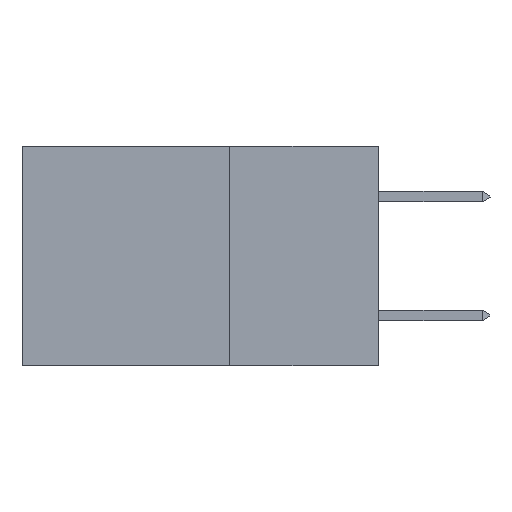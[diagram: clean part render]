
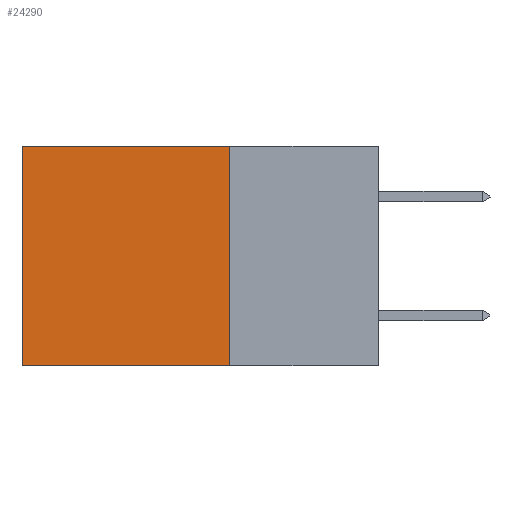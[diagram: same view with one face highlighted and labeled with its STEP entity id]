
A CAD part, left-side view. The second image highlights one B-rep face of the part: STEP entity #24290.
In plain terms, the highlighted planar face has unit normal (-1, 0, 0).
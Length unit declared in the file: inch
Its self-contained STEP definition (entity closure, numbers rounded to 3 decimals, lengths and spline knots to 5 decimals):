
#78 = DIRECTION ( 'NONE',  ( 0., 0., -1. ) ) ;
#156 = DIRECTION ( 'NONE',  ( 0., 1., 0. ) ) ;
#279 = CARTESIAN_POINT ( 'NONE',  ( 0.2615, 0.25, 0. ) ) ;
#519 = ORIENTED_EDGE ( 'NONE', *, *, #6184, .F. ) ;
#1173 = DIRECTION ( 'NONE',  ( 1., 0., 0. ) ) ;
#1572 = DIRECTION ( 'NONE',  ( 0., 0., -1. ) ) ;
#2454 = VERTEX_POINT ( 'NONE', #24584 ) ;
#2591 = LINE ( 'NONE', #279, #8111 ) ;
#3742 = VERTEX_POINT ( 'NONE', #22301 ) ;
#3916 = VECTOR ( 'NONE', #78, 39.37008 ) ;
#4180 = EDGE_CURVE ( 'NONE', #2454, #22378, #2591, .T. ) ;
#4391 = VECTOR ( 'NONE', #25727, 39.37008 ) ;
#6157 = EDGE_LOOP ( 'NONE', ( #12479, #519, #14023, #16129 ) ) ;
#6184 = EDGE_CURVE ( 'NONE', #3742, #22983, #26255, .T. ) ;
#8111 = VECTOR ( 'NONE', #156, 39.37008 ) ;
#10428 = CARTESIAN_POINT ( 'NONE',  ( 0.2615, 0.25, -0.37 ) ) ;
#10721 = LINE ( 'NONE', #10428, #3916 ) ;
#12479 = ORIENTED_EDGE ( 'NONE', *, *, #23753, .T. ) ;
#13534 = CARTESIAN_POINT ( 'NONE',  ( 0.2615, 0.25, -0.37 ) ) ;
#14023 = ORIENTED_EDGE ( 'NONE', *, *, #15324, .F. ) ;
#15324 = EDGE_CURVE ( 'NONE', #2454, #3742, #10721, .T. ) ;
#15607 = DIRECTION ( 'NONE',  ( 0., 0., -1. ) ) ;
#16129 = ORIENTED_EDGE ( 'NONE', *, *, #4180, .T. ) ;
#17507 = AXIS2_PLACEMENT_3D ( 'NONE', #13534, #1173, #15607 ) ;
#17994 = CARTESIAN_POINT ( 'NONE',  ( 0.2615, 0.6, -0.37 ) ) ;
#18664 = LINE ( 'NONE', #20087, #23443 ) ;
#20087 = CARTESIAN_POINT ( 'NONE',  ( 0.2615, 0.6, -0.37 ) ) ;
#21663 = PLANE ( 'NONE',  #17507 ) ;
#22301 = CARTESIAN_POINT ( 'NONE',  ( 0.2615, 0.25, -0.37 ) ) ;
#22378 = VERTEX_POINT ( 'NONE', #25177 ) ;
#22983 = VERTEX_POINT ( 'NONE', #17994 ) ;
#23443 = VECTOR ( 'NONE', #1572, 39.37008 ) ;
#23753 = EDGE_CURVE ( 'NONE', #22378, #22983, #18664, .T. ) ;
#24290 = ADVANCED_FACE ( 'NONE', ( #26329 ), #21663, .F. ) ;
#24584 = CARTESIAN_POINT ( 'NONE',  ( 0.2615, 0.25, 0. ) ) ;
#25177 = CARTESIAN_POINT ( 'NONE',  ( 0.2615, 0.6, 0. ) ) ;
#25727 = DIRECTION ( 'NONE',  ( 0., 1., 0. ) ) ;
#26097 = CARTESIAN_POINT ( 'NONE',  ( 0.2615, 0.25, -0.37 ) ) ;
#26255 = LINE ( 'NONE', #26097, #4391 ) ;
#26329 = FACE_OUTER_BOUND ( 'NONE', #6157, .T. ) ;
